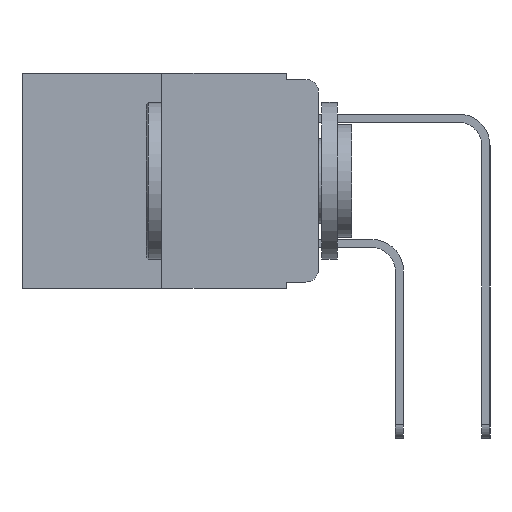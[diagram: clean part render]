
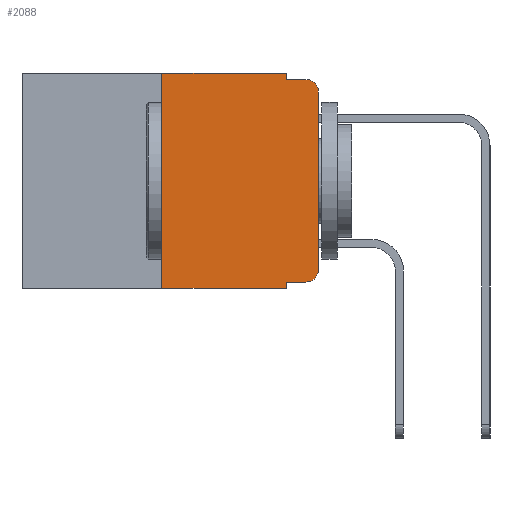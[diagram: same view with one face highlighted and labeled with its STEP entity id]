
A CAD part, left-side view. The second image highlights one B-rep face of the part: STEP entity #2088.
In plain terms, the highlighted planar face has unit normal (-1, 0, 0).
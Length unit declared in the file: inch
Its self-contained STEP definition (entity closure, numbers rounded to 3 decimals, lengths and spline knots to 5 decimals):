
#325 = CARTESIAN_POINT ( 'NONE',  ( 0., 0.051, 0. ) ) ;
#466 = CARTESIAN_POINT ( 'NONE',  ( 0., 0.051, 0. ) ) ;
#720 = VERTEX_POINT ( 'NONE', #19233 ) ;
#843 = CIRCLE ( 'NONE', #8645, 0.02 ) ;
#1525 = DIRECTION ( 'NONE',  ( 0., -1., 0. ) ) ;
#1789 = EDGE_CURVE ( 'NONE', #12195, #720, #5089, .T. ) ;
#1844 = EDGE_CURVE ( 'NONE', #18504, #6997, #16589, .T. ) ;
#2088 = ADVANCED_FACE ( 'NONE', ( #12229 ), #6707, .F. ) ;
#2377 = CARTESIAN_POINT ( 'NONE',  ( 0., 0., -0.313 ) ) ;
#2588 = CARTESIAN_POINT ( 'NONE',  ( 0., 0.02, -0.313 ) ) ;
#2790 = CARTESIAN_POINT ( 'NONE',  ( 0., 0.02, -0.01 ) ) ;
#2812 = VERTEX_POINT ( 'NONE', #8960 ) ;
#2904 = VECTOR ( 'NONE', #1525, 39.37008 ) ;
#3246 = ORIENTED_EDGE ( 'NONE', *, *, #1789, .T. ) ;
#3536 = VECTOR ( 'NONE', #4621, 39.37008 ) ;
#3578 = DIRECTION ( 'NONE',  ( 0., 0., 1. ) ) ;
#3785 = CARTESIAN_POINT ( 'NONE',  ( 0., 0.02, -0.03 ) ) ;
#3846 = DIRECTION ( 'NONE',  ( 0., -1., 0. ) ) ;
#4236 = DIRECTION ( 'NONE',  ( 0., 0., -1. ) ) ;
#4250 = ORIENTED_EDGE ( 'NONE', *, *, #17385, .T. ) ;
#4527 = CARTESIAN_POINT ( 'NONE',  ( 0., 0.25, 0. ) ) ;
#4621 = DIRECTION ( 'NONE',  ( 0., -1., 0. ) ) ;
#5015 = CIRCLE ( 'NONE', #5496, 0.02 ) ;
#5042 = ORIENTED_EDGE ( 'NONE', *, *, #5499, .T. ) ;
#5089 = LINE ( 'NONE', #8647, #17075 ) ;
#5262 = DIRECTION ( 'NONE',  ( 0., 0., -1. ) ) ;
#5407 = DIRECTION ( 'NONE',  ( 0., 0., -1. ) ) ;
#5496 = AXIS2_PLACEMENT_3D ( 'NONE', #2588, #13728, #4236 ) ;
#5499 = EDGE_CURVE ( 'NONE', #6828, #7234, #18440, .T. ) ;
#6010 = EDGE_CURVE ( 'NONE', #2812, #6828, #5015, .T. ) ;
#6018 = ORIENTED_EDGE ( 'NONE', *, *, #10962, .F. ) ;
#6370 = VERTEX_POINT ( 'NONE', #12582 ) ;
#6526 = ORIENTED_EDGE ( 'NONE', *, *, #10068, .F. ) ;
#6707 = PLANE ( 'NONE',  #20294 ) ;
#6791 = DIRECTION ( 'NONE',  ( 0., 0., -1. ) ) ;
#6828 = VERTEX_POINT ( 'NONE', #2377 ) ;
#6881 = DIRECTION ( 'NONE',  ( 1., 0., 0. ) ) ;
#6997 = VERTEX_POINT ( 'NONE', #2790 ) ;
#7084 = EDGE_LOOP ( 'NONE', ( #5042, #17509, #9728, #6018, #6526, #14854, #3246, #7981, #4250, #16783 ) ) ;
#7234 = VERTEX_POINT ( 'NONE', #14571 ) ;
#7375 = VECTOR ( 'NONE', #5262, 39.37008 ) ;
#7873 = DIRECTION ( 'NONE',  ( 0., -1., 0. ) ) ;
#7981 = ORIENTED_EDGE ( 'NONE', *, *, #8488, .F. ) ;
#8488 = EDGE_CURVE ( 'NONE', #6370, #720, #15229, .T. ) ;
#8522 = LINE ( 'NONE', #19887, #11232 ) ;
#8645 = AXIS2_PLACEMENT_3D ( 'NONE', #3785, #14812, #5407 ) ;
#8647 = CARTESIAN_POINT ( 'NONE',  ( 0., 0.473, -0.343 ) ) ;
#8960 = CARTESIAN_POINT ( 'NONE',  ( 0., 0.02, -0.333 ) ) ;
#9059 = DIRECTION ( 'NONE',  ( 0., 0., -1. ) ) ;
#9728 = ORIENTED_EDGE ( 'NONE', *, *, #1844, .F. ) ;
#10068 = EDGE_CURVE ( 'NONE', #19049, #11453, #12268, .T. ) ;
#10916 = CARTESIAN_POINT ( 'NONE',  ( 0., 0.473, 0. ) ) ;
#10962 = EDGE_CURVE ( 'NONE', #11453, #18504, #8522, .T. ) ;
#11232 = VECTOR ( 'NONE', #9059, 39.37008 ) ;
#11453 = VERTEX_POINT ( 'NONE', #466 ) ;
#11760 = CARTESIAN_POINT ( 'NONE',  ( 0., 0.473, 0. ) ) ;
#11840 = LINE ( 'NONE', #13101, #16437 ) ;
#12027 = DIRECTION ( 'NONE',  ( 0., 0., 1. ) ) ;
#12195 = VERTEX_POINT ( 'NONE', #18069 ) ;
#12229 = FACE_OUTER_BOUND ( 'NONE', #7084, .T. ) ;
#12268 = LINE ( 'NONE', #11760, #15905 ) ;
#12582 = CARTESIAN_POINT ( 'NONE',  ( 0., 0.051, -0.333 ) ) ;
#12719 = CARTESIAN_POINT ( 'NONE',  ( 0., 0.051, -0.333 ) ) ;
#13101 = CARTESIAN_POINT ( 'NONE',  ( 0., 0.25, 0. ) ) ;
#13456 = EDGE_CURVE ( 'NONE', #7234, #6997, #843, .T. ) ;
#13728 = DIRECTION ( 'NONE',  ( -1., 0., 0. ) ) ;
#14373 = VECTOR ( 'NONE', #12027, 39.37008 ) ;
#14549 = LINE ( 'NONE', #12719, #2904 ) ;
#14571 = CARTESIAN_POINT ( 'NONE',  ( 0., 0., -0.03 ) ) ;
#14812 = DIRECTION ( 'NONE',  ( -1., 0., 0. ) ) ;
#14854 = ORIENTED_EDGE ( 'NONE', *, *, #19762, .F. ) ;
#15229 = LINE ( 'NONE', #325, #7375 ) ;
#15905 = VECTOR ( 'NONE', #3846, 39.37008 ) ;
#16437 = VECTOR ( 'NONE', #3578, 39.37008 ) ;
#16589 = LINE ( 'NONE', #20153, #3536 ) ;
#16783 = ORIENTED_EDGE ( 'NONE', *, *, #6010, .T. ) ;
#17075 = VECTOR ( 'NONE', #7873, 39.37008 ) ;
#17385 = EDGE_CURVE ( 'NONE', #6370, #2812, #14549, .T. ) ;
#17509 = ORIENTED_EDGE ( 'NONE', *, *, #13456, .T. ) ;
#18069 = CARTESIAN_POINT ( 'NONE',  ( 0., 0.25, -0.343 ) ) ;
#18151 = CARTESIAN_POINT ( 'NONE',  ( 0., 0., 0. ) ) ;
#18440 = LINE ( 'NONE', #18151, #14373 ) ;
#18504 = VERTEX_POINT ( 'NONE', #19994 ) ;
#19049 = VERTEX_POINT ( 'NONE', #4527 ) ;
#19233 = CARTESIAN_POINT ( 'NONE',  ( 0., 0.051, -0.343 ) ) ;
#19762 = EDGE_CURVE ( 'NONE', #12195, #19049, #11840, .T. ) ;
#19887 = CARTESIAN_POINT ( 'NONE',  ( 0., 0.051, 0. ) ) ;
#19994 = CARTESIAN_POINT ( 'NONE',  ( 0., 0.051, -0.01 ) ) ;
#20153 = CARTESIAN_POINT ( 'NONE',  ( 0., 0.051, -0.01 ) ) ;
#20294 = AXIS2_PLACEMENT_3D ( 'NONE', #10916, #6881, #6791 ) ;
